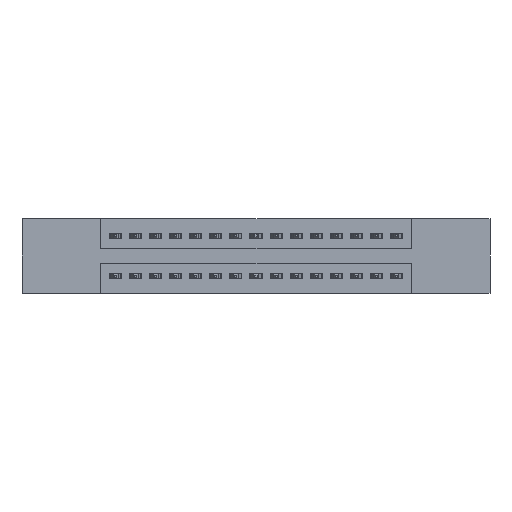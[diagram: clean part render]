
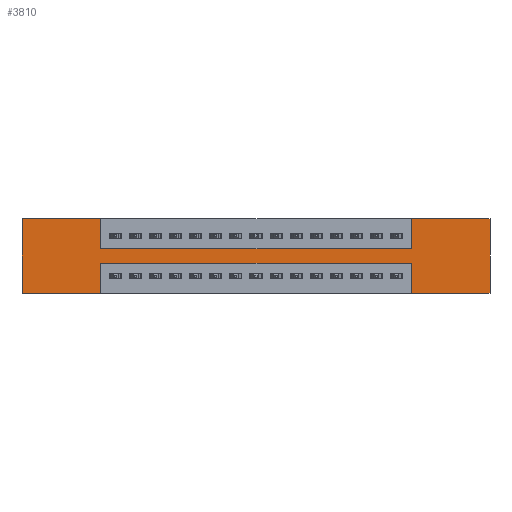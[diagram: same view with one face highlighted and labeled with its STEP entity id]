
A CAD part, front view. The second image highlights one B-rep face of the part: STEP entity #3810.
In plain terms, the highlighted planar face has unit normal (0, -1, 0).
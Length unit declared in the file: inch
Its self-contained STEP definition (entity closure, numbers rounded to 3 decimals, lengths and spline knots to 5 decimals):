
#53 = VECTOR ( 'NONE', #423, 39.37008 ) ;
#62 = AXIS2_PLACEMENT_3D ( 'NONE', #9409, #8204, #15159 ) ;
#423 = DIRECTION ( 'NONE',  ( -1., 0., 0. ) ) ;
#445 = CARTESIAN_POINT ( 'NONE',  ( 1.9425, 0., -0.37 ) ) ;
#453 = ORIENTED_EDGE ( 'NONE', *, *, #1329, .F. ) ;
#950 = CARTESIAN_POINT ( 'NONE',  ( 0.3925, 0., -0.37 ) ) ;
#1329 = EDGE_CURVE ( 'NONE', #2612, #10634, #13573, .T. ) ;
#1432 = CARTESIAN_POINT ( 'NONE',  ( 0.3925, 0., 0. ) ) ;
#1815 = LINE ( 'NONE', #1972, #4668 ) ;
#1962 = VERTEX_POINT ( 'NONE', #5528 ) ;
#1972 = CARTESIAN_POINT ( 'NONE',  ( 0., 0., -0.37 ) ) ;
#2103 = VERTEX_POINT ( 'NONE', #7205 ) ;
#2130 = VERTEX_POINT ( 'NONE', #2783 ) ;
#2209 = PLANE ( 'NONE',  #62 ) ;
#2261 = EDGE_CURVE ( 'NONE', #6030, #2797, #12119, .T. ) ;
#2273 = VERTEX_POINT ( 'NONE', #1432 ) ;
#2369 = EDGE_CURVE ( 'NONE', #2797, #10703, #10651, .T. ) ;
#2475 = LINE ( 'NONE', #13673, #15023 ) ;
#2612 = VERTEX_POINT ( 'NONE', #4747 ) ;
#2748 = CARTESIAN_POINT ( 'NONE',  ( 1.9425, 0., -0.15 ) ) ;
#2783 = CARTESIAN_POINT ( 'NONE',  ( 0., 0., 0. ) ) ;
#2797 = VERTEX_POINT ( 'NONE', #5196 ) ;
#3490 = VECTOR ( 'NONE', #7401, 39.37008 ) ;
#3675 = LINE ( 'NONE', #11557, #8925 ) ;
#3723 = ORIENTED_EDGE ( 'NONE', *, *, #10507, .F. ) ;
#3810 = ADVANCED_FACE ( 'NONE', ( #9871 ), #2209, .T. ) ;
#4090 = EDGE_CURVE ( 'NONE', #1962, #2130, #9144, .T. ) ;
#4220 = CARTESIAN_POINT ( 'NONE',  ( 1.9425, 0., -0.37 ) ) ;
#4229 = EDGE_LOOP ( 'NONE', ( #4294, #453, #3723, #5624, #10363, #7207, #8578, #4964, #13287, #10572, #4613, #4978 ) ) ;
#4294 = ORIENTED_EDGE ( 'NONE', *, *, #10790, .F. ) ;
#4387 = DIRECTION ( 'NONE',  ( 1., 0., 0. ) ) ;
#4613 = ORIENTED_EDGE ( 'NONE', *, *, #4090, .F. ) ;
#4668 = VECTOR ( 'NONE', #11543, 39.37008 ) ;
#4747 = CARTESIAN_POINT ( 'NONE',  ( 1.9425, 0., -0.22 ) ) ;
#4964 = ORIENTED_EDGE ( 'NONE', *, *, #7807, .F. ) ;
#4978 = ORIENTED_EDGE ( 'NONE', *, *, #12164, .F. ) ;
#5112 = EDGE_CURVE ( 'NONE', #2130, #2273, #3675, .T. ) ;
#5196 = CARTESIAN_POINT ( 'NONE',  ( 1.9425, 0., 0. ) ) ;
#5223 = VECTOR ( 'NONE', #14232, 39.37008 ) ;
#5363 = CARTESIAN_POINT ( 'NONE',  ( 0., 0., 0. ) ) ;
#5528 = CARTESIAN_POINT ( 'NONE',  ( 0., 0., -0.37 ) ) ;
#5538 = LINE ( 'NONE', #13263, #3490 ) ;
#5624 = ORIENTED_EDGE ( 'NONE', *, *, #11961, .F. ) ;
#5699 = CARTESIAN_POINT ( 'NONE',  ( 2.335, 0., 0. ) ) ;
#6009 = CARTESIAN_POINT ( 'NONE',  ( 0., 0., -0.37 ) ) ;
#6030 = VERTEX_POINT ( 'NONE', #2748 ) ;
#6037 = DIRECTION ( 'NONE',  ( 0., 0., 1. ) ) ;
#6372 = LINE ( 'NONE', #14964, #8413 ) ;
#6573 = VECTOR ( 'NONE', #10154, 39.37008 ) ;
#6579 = CARTESIAN_POINT ( 'NONE',  ( 2.335, 0., -0.37 ) ) ;
#6632 = DIRECTION ( 'NONE',  ( 0., 0., -1. ) ) ;
#6664 = CARTESIAN_POINT ( 'NONE',  ( 0.3925, 0., -0.22 ) ) ;
#7205 = CARTESIAN_POINT ( 'NONE',  ( 0.3925, 0., -0.37 ) ) ;
#7207 = ORIENTED_EDGE ( 'NONE', *, *, #2369, .F. ) ;
#7401 = DIRECTION ( 'NONE',  ( 1., 0., 0. ) ) ;
#7474 = VECTOR ( 'NONE', #11232, 39.37008 ) ;
#7476 = VERTEX_POINT ( 'NONE', #6579 ) ;
#7807 = EDGE_CURVE ( 'NONE', #14457, #6030, #5538, .T. ) ;
#7995 = CARTESIAN_POINT ( 'NONE',  ( 0.3925, 0., -0.22 ) ) ;
#8010 = LINE ( 'NONE', #6009, #5223 ) ;
#8204 = DIRECTION ( 'NONE',  ( 0., -1., 0. ) ) ;
#8413 = VECTOR ( 'NONE', #10388, 39.37008 ) ;
#8578 = ORIENTED_EDGE ( 'NONE', *, *, #2261, .F. ) ;
#8832 = VECTOR ( 'NONE', #14078, 39.37008 ) ;
#8925 = VECTOR ( 'NONE', #4387, 39.37008 ) ;
#8998 = VECTOR ( 'NONE', #10050, 39.37008 ) ;
#9144 = LINE ( 'NONE', #15400, #9510 ) ;
#9398 = EDGE_CURVE ( 'NONE', #10703, #7476, #2475, .T. ) ;
#9409 = CARTESIAN_POINT ( 'NONE',  ( 0., 0., -0.37 ) ) ;
#9510 = VECTOR ( 'NONE', #6037, 39.37008 ) ;
#9756 = LINE ( 'NONE', #445, #6573 ) ;
#9871 = FACE_OUTER_BOUND ( 'NONE', #4229, .T. ) ;
#10050 = DIRECTION ( 'NONE',  ( 0., 0., 1. ) ) ;
#10154 = DIRECTION ( 'NONE',  ( 0., 0., 1. ) ) ;
#10363 = ORIENTED_EDGE ( 'NONE', *, *, #9398, .F. ) ;
#10388 = DIRECTION ( 'NONE',  ( 0., 0., -1. ) ) ;
#10507 = EDGE_CURVE ( 'NONE', #14394, #2612, #9756, .T. ) ;
#10572 = ORIENTED_EDGE ( 'NONE', *, *, #5112, .F. ) ;
#10634 = VERTEX_POINT ( 'NONE', #7995 ) ;
#10651 = LINE ( 'NONE', #5363, #7474 ) ;
#10703 = VERTEX_POINT ( 'NONE', #5699 ) ;
#10790 = EDGE_CURVE ( 'NONE', #10634, #2103, #15330, .T. ) ;
#11232 = DIRECTION ( 'NONE',  ( 1., 0., 0. ) ) ;
#11267 = EDGE_CURVE ( 'NONE', #2273, #14457, #6372, .T. ) ;
#11424 = CARTESIAN_POINT ( 'NONE',  ( 1.9425, 0., 0. ) ) ;
#11543 = DIRECTION ( 'NONE',  ( -1., 0., 0. ) ) ;
#11557 = CARTESIAN_POINT ( 'NONE',  ( 0., 0., 0. ) ) ;
#11961 = EDGE_CURVE ( 'NONE', #7476, #14394, #1815, .T. ) ;
#12119 = LINE ( 'NONE', #11424, #8998 ) ;
#12164 = EDGE_CURVE ( 'NONE', #2103, #1962, #8010, .T. ) ;
#12661 = CARTESIAN_POINT ( 'NONE',  ( 0.3925, 0., -0.15 ) ) ;
#13263 = CARTESIAN_POINT ( 'NONE',  ( 0.3925, 0., -0.15 ) ) ;
#13287 = ORIENTED_EDGE ( 'NONE', *, *, #11267, .F. ) ;
#13573 = LINE ( 'NONE', #6664, #53 ) ;
#13673 = CARTESIAN_POINT ( 'NONE',  ( 2.335, 0., 0. ) ) ;
#14078 = DIRECTION ( 'NONE',  ( 0., 0., -1. ) ) ;
#14232 = DIRECTION ( 'NONE',  ( -1., 0., 0. ) ) ;
#14394 = VERTEX_POINT ( 'NONE', #4220 ) ;
#14457 = VERTEX_POINT ( 'NONE', #12661 ) ;
#14964 = CARTESIAN_POINT ( 'NONE',  ( 0.3925, 0., 0. ) ) ;
#15023 = VECTOR ( 'NONE', #6632, 39.37008 ) ;
#15159 = DIRECTION ( 'NONE',  ( 0., 0., -1. ) ) ;
#15330 = LINE ( 'NONE', #950, #8832 ) ;
#15400 = CARTESIAN_POINT ( 'NONE',  ( 0., 0., 0. ) ) ;
